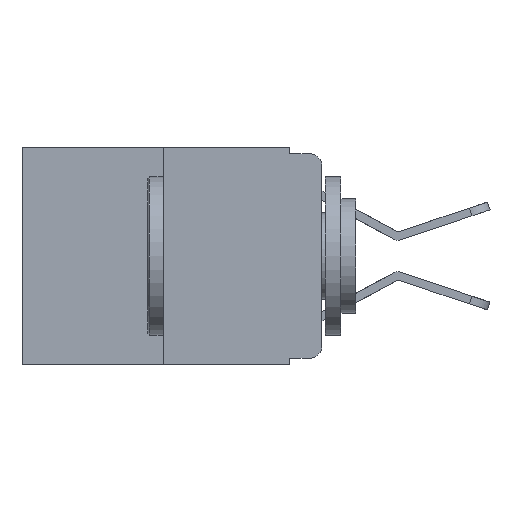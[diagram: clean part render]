
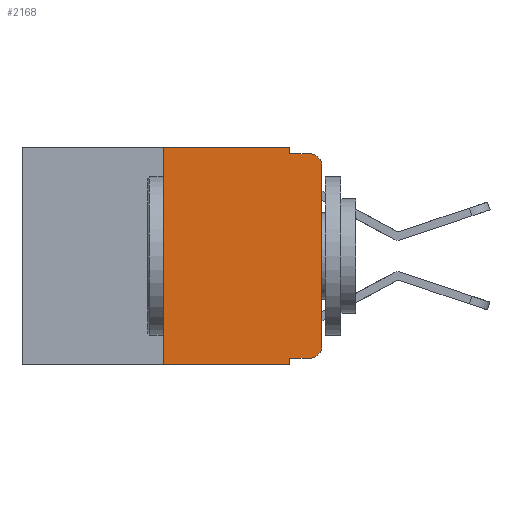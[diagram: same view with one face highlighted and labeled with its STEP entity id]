
A CAD part, left-side view. The second image highlights one B-rep face of the part: STEP entity #2168.
In plain terms, the highlighted planar face has unit normal (-1, 0, 0).
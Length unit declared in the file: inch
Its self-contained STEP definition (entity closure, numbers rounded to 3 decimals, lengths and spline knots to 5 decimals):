
#102 = EDGE_CURVE ( 'NONE', #9237, #2246, #19816, .T. ) ;
#282 = EDGE_CURVE ( 'NONE', #14299, #18607, #4924, .T. ) ;
#509 = CIRCLE ( 'NONE', #10133, 0.02 ) ;
#626 = ORIENTED_EDGE ( 'NONE', *, *, #6254, .T. ) ;
#891 = EDGE_CURVE ( 'NONE', #2623, #4015, #9441, .T. ) ;
#1019 = ORIENTED_EDGE ( 'NONE', *, *, #2216, .T. ) ;
#1453 = VECTOR ( 'NONE', #12997, 39.37008 ) ;
#1692 = CARTESIAN_POINT ( 'NONE',  ( 0., 0.051, 0. ) ) ;
#1764 = CARTESIAN_POINT ( 'NONE',  ( 0., 0.473, -0.343 ) ) ;
#1844 = DIRECTION ( 'NONE',  ( 0., 0., 1. ) ) ;
#2168 = ADVANCED_FACE ( 'NONE', ( #5603 ), #18347, .F. ) ;
#2210 = DIRECTION ( 'NONE',  ( 0., 0., -1. ) ) ;
#2216 = EDGE_CURVE ( 'NONE', #4015, #6220, #4919, .T. ) ;
#2246 = VERTEX_POINT ( 'NONE', #20128 ) ;
#2374 = DIRECTION ( 'NONE',  ( 0., 0., -1. ) ) ;
#2623 = VERTEX_POINT ( 'NONE', #4333 ) ;
#3302 = CARTESIAN_POINT ( 'NONE',  ( 0., 0.02, -0.01 ) ) ;
#3571 = ORIENTED_EDGE ( 'NONE', *, *, #9602, .T. ) ;
#3675 = VERTEX_POINT ( 'NONE', #20278 ) ;
#3925 = VERTEX_POINT ( 'NONE', #5310 ) ;
#4015 = VERTEX_POINT ( 'NONE', #6878 ) ;
#4333 = CARTESIAN_POINT ( 'NONE',  ( 0., 0., -0.313 ) ) ;
#4538 = VECTOR ( 'NONE', #20348, 39.37008 ) ;
#4558 = CARTESIAN_POINT ( 'NONE',  ( 0., 0.02, -0.03 ) ) ;
#4919 = CIRCLE ( 'NONE', #5276, 0.02 ) ;
#4924 = LINE ( 'NONE', #11286, #10494 ) ;
#4959 = CARTESIAN_POINT ( 'NONE',  ( 0., 0.25, 0. ) ) ;
#5019 = DIRECTION ( 'NONE',  ( 0., -1., 0. ) ) ;
#5141 = AXIS2_PLACEMENT_3D ( 'NONE', #14680, #6750, #13124 ) ;
#5276 = AXIS2_PLACEMENT_3D ( 'NONE', #4558, #7474, #7374 ) ;
#5310 = CARTESIAN_POINT ( 'NONE',  ( 0., 0.051, -0.01 ) ) ;
#5580 = ORIENTED_EDGE ( 'NONE', *, *, #11973, .F. ) ;
#5603 = FACE_OUTER_BOUND ( 'NONE', #9961, .T. ) ;
#6124 = CARTESIAN_POINT ( 'NONE',  ( 0., 0.051, -0.01 ) ) ;
#6220 = VERTEX_POINT ( 'NONE', #3302 ) ;
#6254 = EDGE_CURVE ( 'NONE', #3675, #2246, #17911, .T. ) ;
#6748 = EDGE_CURVE ( 'NONE', #3925, #6220, #12497, .T. ) ;
#6750 = DIRECTION ( 'NONE',  ( 1., 0., 0. ) ) ;
#6878 = CARTESIAN_POINT ( 'NONE',  ( 0., 0., -0.03 ) ) ;
#6921 = LINE ( 'NONE', #17618, #12571 ) ;
#7083 = ORIENTED_EDGE ( 'NONE', *, *, #891, .T. ) ;
#7115 = VECTOR ( 'NONE', #1844, 39.37008 ) ;
#7374 = DIRECTION ( 'NONE',  ( 0., 0., -1. ) ) ;
#7474 = DIRECTION ( 'NONE',  ( -1., 0., 0. ) ) ;
#8013 = DIRECTION ( 'NONE',  ( 0., -1., 0. ) ) ;
#8021 = ORIENTED_EDGE ( 'NONE', *, *, #15289, .F. ) ;
#9237 = VERTEX_POINT ( 'NONE', #19894 ) ;
#9340 = CARTESIAN_POINT ( 'NONE',  ( 0., 0., 0. ) ) ;
#9402 = CARTESIAN_POINT ( 'NONE',  ( 0., 0.25, 0. ) ) ;
#9441 = LINE ( 'NONE', #9340, #7115 ) ;
#9602 = EDGE_CURVE ( 'NONE', #17747, #2623, #509, .T. ) ;
#9961 = EDGE_LOOP ( 'NONE', ( #7083, #1019, #19144, #5580, #13207, #8021, #626, #18562, #20147, #3571 ) ) ;
#10133 = AXIS2_PLACEMENT_3D ( 'NONE', #19673, #13491, #2374 ) ;
#10257 = DIRECTION ( 'NONE',  ( 0., -1., 0. ) ) ;
#10494 = VECTOR ( 'NONE', #5019, 39.37008 ) ;
#11286 = CARTESIAN_POINT ( 'NONE',  ( 0., 0.473, 0. ) ) ;
#11508 = LINE ( 'NONE', #4959, #16260 ) ;
#11765 = CARTESIAN_POINT ( 'NONE',  ( 0., 0.051, 0. ) ) ;
#11973 = EDGE_CURVE ( 'NONE', #18607, #3925, #12506, .T. ) ;
#12001 = CARTESIAN_POINT ( 'NONE',  ( 0., 0.02, -0.333 ) ) ;
#12204 = VECTOR ( 'NONE', #2210, 39.37008 ) ;
#12497 = LINE ( 'NONE', #6124, #16424 ) ;
#12506 = LINE ( 'NONE', #1692, #4538 ) ;
#12571 = VECTOR ( 'NONE', #10257, 39.37008 ) ;
#12997 = DIRECTION ( 'NONE',  ( 0., -1., 0. ) ) ;
#13124 = DIRECTION ( 'NONE',  ( 0., 0., -1. ) ) ;
#13207 = ORIENTED_EDGE ( 'NONE', *, *, #282, .F. ) ;
#13491 = DIRECTION ( 'NONE',  ( -1., 0., 0. ) ) ;
#14299 = VERTEX_POINT ( 'NONE', #9402 ) ;
#14680 = CARTESIAN_POINT ( 'NONE',  ( 0., 0.473, 0. ) ) ;
#15289 = EDGE_CURVE ( 'NONE', #3675, #14299, #11508, .T. ) ;
#16260 = VECTOR ( 'NONE', #17705, 39.37008 ) ;
#16424 = VECTOR ( 'NONE', #8013, 39.37008 ) ;
#17618 = CARTESIAN_POINT ( 'NONE',  ( 0., 0.051, -0.333 ) ) ;
#17705 = DIRECTION ( 'NONE',  ( 0., 0., 1. ) ) ;
#17747 = VERTEX_POINT ( 'NONE', #12001 ) ;
#17911 = LINE ( 'NONE', #1764, #1453 ) ;
#18347 = PLANE ( 'NONE',  #5141 ) ;
#18562 = ORIENTED_EDGE ( 'NONE', *, *, #102, .F. ) ;
#18607 = VERTEX_POINT ( 'NONE', #20177 ) ;
#19144 = ORIENTED_EDGE ( 'NONE', *, *, #6748, .F. ) ;
#19646 = EDGE_CURVE ( 'NONE', #9237, #17747, #6921, .T. ) ;
#19673 = CARTESIAN_POINT ( 'NONE',  ( 0., 0.02, -0.313 ) ) ;
#19816 = LINE ( 'NONE', #11765, #12204 ) ;
#19894 = CARTESIAN_POINT ( 'NONE',  ( 0., 0.051, -0.333 ) ) ;
#20128 = CARTESIAN_POINT ( 'NONE',  ( 0., 0.051, -0.343 ) ) ;
#20147 = ORIENTED_EDGE ( 'NONE', *, *, #19646, .T. ) ;
#20177 = CARTESIAN_POINT ( 'NONE',  ( 0., 0.051, 0. ) ) ;
#20278 = CARTESIAN_POINT ( 'NONE',  ( 0., 0.25, -0.343 ) ) ;
#20348 = DIRECTION ( 'NONE',  ( 0., 0., -1. ) ) ;
